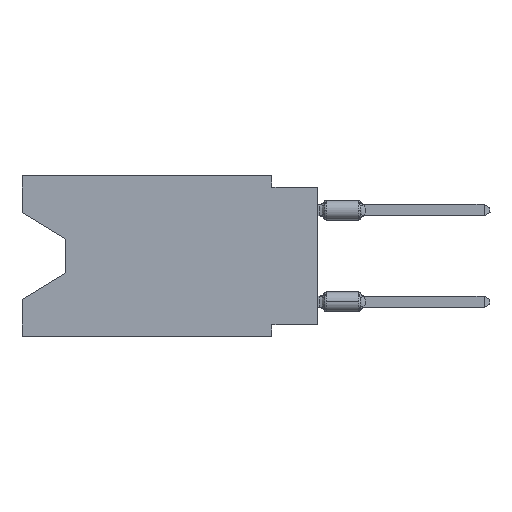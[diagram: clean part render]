
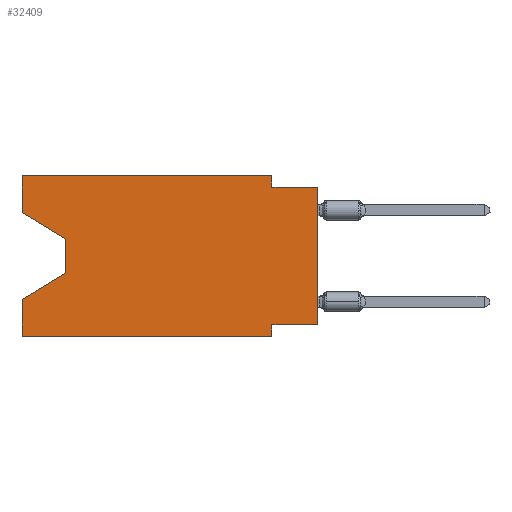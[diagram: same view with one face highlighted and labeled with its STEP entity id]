
A CAD part, left-side view. The second image highlights one B-rep face of the part: STEP entity #32409.
In plain terms, the highlighted planar face has unit normal (-1, 0, 0).
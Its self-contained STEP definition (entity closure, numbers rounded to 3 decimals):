
#1555 = VECTOR ( 'NONE', #13114, 1000. ) ;
#2127 = EDGE_CURVE ( 'NONE', #6122, #20296, #10588, .T. ) ;
#2424 = VECTOR ( 'NONE', #17949, 1000. ) ;
#2964 = ORIENTED_EDGE ( 'NONE', *, *, #2127, .T. ) ;
#3343 = CARTESIAN_POINT ( 'NONE',  ( 0., 16.383, 0. ) ) ;
#3591 = LINE ( 'NONE', #17284, #8170 ) ;
#3980 = EDGE_CURVE ( 'NONE', #21906, #12121, #20097, .T. ) ;
#5154 = VERTEX_POINT ( 'NONE', #24894 ) ;
#5401 = LINE ( 'NONE', #36167, #9045 ) ;
#5433 = ORIENTED_EDGE ( 'NONE', *, *, #13943, .T. ) ;
#6122 = VERTEX_POINT ( 'NONE', #23153 ) ;
#6613 = CARTESIAN_POINT ( 'NONE',  ( 0., 16.383, 0. ) ) ;
#7440 = DIRECTION ( 'NONE',  ( 0., -0.855, -0.519 ) ) ;
#7630 = VERTEX_POINT ( 'NONE', #41982 ) ;
#8170 = VECTOR ( 'NONE', #9881, 1000. ) ;
#8383 = CARTESIAN_POINT ( 'NONE',  ( 0., 13.97, -3.505 ) ) ;
#8502 = CARTESIAN_POINT ( 'NONE',  ( 0., 2.54, 0. ) ) ;
#9045 = VECTOR ( 'NONE', #22942, 1000. ) ;
#9091 = EDGE_CURVE ( 'NONE', #21906, #24335, #5401, .T. ) ;
#9234 = EDGE_LOOP ( 'NONE', ( #2964, #10664, #5433, #18871, #29404, #34020, #12532, #31172, #17175, #41282, #22954, #24127 ) ) ;
#9881 = DIRECTION ( 'NONE',  ( 0., -1., 0. ) ) ;
#10588 = LINE ( 'NONE', #38016, #40157 ) ;
#10664 = ORIENTED_EDGE ( 'NONE', *, *, #19713, .T. ) ;
#10834 = CARTESIAN_POINT ( 'NONE',  ( 0., 2.54, -8.255 ) ) ;
#10869 = AXIS2_PLACEMENT_3D ( 'NONE', #35671, #14783, #24690 ) ;
#11418 = FACE_OUTER_BOUND ( 'NONE', #9234, .T. ) ;
#11859 = DIRECTION ( 'NONE',  ( 0., 0., -1. ) ) ;
#12121 = VERTEX_POINT ( 'NONE', #19804 ) ;
#12532 = ORIENTED_EDGE ( 'NONE', *, *, #29474, .F. ) ;
#13114 = DIRECTION ( 'NONE',  ( 0., 0., 1. ) ) ;
#13943 = EDGE_CURVE ( 'NONE', #25953, #12121, #14110, .T. ) ;
#14110 = LINE ( 'NONE', #28056, #43841 ) ;
#14356 = LINE ( 'NONE', #28064, #2424 ) ;
#14604 = LINE ( 'NONE', #23880, #28732 ) ;
#14783 = DIRECTION ( 'NONE',  ( 1., 0., 0. ) ) ;
#14991 = VECTOR ( 'NONE', #36003, 1000. ) ;
#16098 = VECTOR ( 'NONE', #30619, 1000. ) ;
#17175 = ORIENTED_EDGE ( 'NONE', *, *, #29355, .F. ) ;
#17284 = CARTESIAN_POINT ( 'NONE',  ( 0., 0., -0.635 ) ) ;
#17919 = VERTEX_POINT ( 'NONE', #44196 ) ;
#17949 = DIRECTION ( 'NONE',  ( 0., 1., 0. ) ) ;
#18482 = LINE ( 'NONE', #8383, #14991 ) ;
#18871 = ORIENTED_EDGE ( 'NONE', *, *, #3980, .F. ) ;
#19713 = EDGE_CURVE ( 'NONE', #20296, #25953, #18482, .T. ) ;
#19804 = CARTESIAN_POINT ( 'NONE',  ( 0., 16.383, -6.852 ) ) ;
#20097 = LINE ( 'NONE', #6613, #1555 ) ;
#20296 = VERTEX_POINT ( 'NONE', #43381 ) ;
#20434 = LINE ( 'NONE', #3343, #37351 ) ;
#21488 = DIRECTION ( 'NONE',  ( 0., 0., 1. ) ) ;
#21906 = VERTEX_POINT ( 'NONE', #28738 ) ;
#22920 = EDGE_CURVE ( 'NONE', #6122, #33546, #14604, .T. ) ;
#22942 = DIRECTION ( 'NONE',  ( 0., -1., 0. ) ) ;
#22954 = ORIENTED_EDGE ( 'NONE', *, *, #23321, .F. ) ;
#23084 = VECTOR ( 'NONE', #21488, 1000. ) ;
#23153 = CARTESIAN_POINT ( 'NONE',  ( 0., 16.383, -2.038 ) ) ;
#23222 = CARTESIAN_POINT ( 'NONE',  ( 0., 16.383, 0. ) ) ;
#23321 = EDGE_CURVE ( 'NONE', #33546, #30967, #20434, .T. ) ;
#23689 = CARTESIAN_POINT ( 'NONE',  ( 0., 2.54, -8.89 ) ) ;
#23880 = CARTESIAN_POINT ( 'NONE',  ( 0., 16.383, 0. ) ) ;
#24127 = ORIENTED_EDGE ( 'NONE', *, *, #22920, .F. ) ;
#24335 = VERTEX_POINT ( 'NONE', #29056 ) ;
#24690 = DIRECTION ( 'NONE',  ( 0., 0., -1. ) ) ;
#24894 = CARTESIAN_POINT ( 'NONE',  ( 0., 0., -0.635 ) ) ;
#25081 = CARTESIAN_POINT ( 'NONE',  ( 0., 0., 0. ) ) ;
#25574 = LINE ( 'NONE', #8502, #38301 ) ;
#25953 = VERTEX_POINT ( 'NONE', #41848 ) ;
#28056 = CARTESIAN_POINT ( 'NONE',  ( 0., 13.97, -5.385 ) ) ;
#28064 = CARTESIAN_POINT ( 'NONE',  ( 0., 0., -8.255 ) ) ;
#28732 = VECTOR ( 'NONE', #42276, 1000. ) ;
#28734 = PLANE ( 'NONE',  #10869 ) ;
#28738 = CARTESIAN_POINT ( 'NONE',  ( 0., 16.383, -8.89 ) ) ;
#29056 = CARTESIAN_POINT ( 'NONE',  ( 0., 2.54, -8.89 ) ) ;
#29355 = EDGE_CURVE ( 'NONE', #7630, #5154, #3591, .T. ) ;
#29404 = ORIENTED_EDGE ( 'NONE', *, *, #9091, .T. ) ;
#29450 = EDGE_CURVE ( 'NONE', #30967, #7630, #25574, .T. ) ;
#29474 = EDGE_CURVE ( 'NONE', #17919, #44167, #14356, .T. ) ;
#30619 = DIRECTION ( 'NONE',  ( 0., 0., -1. ) ) ;
#30967 = VERTEX_POINT ( 'NONE', #43839 ) ;
#30990 = DIRECTION ( 'NONE',  ( 0., 0.855, -0.519 ) ) ;
#31172 = ORIENTED_EDGE ( 'NONE', *, *, #32789, .T. ) ;
#32409 = ADVANCED_FACE ( 'NONE', ( #11418 ), #28734, .F. ) ;
#32789 = EDGE_CURVE ( 'NONE', #17919, #5154, #35384, .T. ) ;
#33546 = VERTEX_POINT ( 'NONE', #23222 ) ;
#34020 = ORIENTED_EDGE ( 'NONE', *, *, #35601, .F. ) ;
#35384 = LINE ( 'NONE', #25081, #23084 ) ;
#35601 = EDGE_CURVE ( 'NONE', #44167, #24335, #40756, .T. ) ;
#35671 = CARTESIAN_POINT ( 'NONE',  ( 0., 16.383, 0. ) ) ;
#36003 = DIRECTION ( 'NONE',  ( 0., 0., -1. ) ) ;
#36167 = CARTESIAN_POINT ( 'NONE',  ( 0., 16.383, -8.89 ) ) ;
#37351 = VECTOR ( 'NONE', #44275, 1000. ) ;
#38016 = CARTESIAN_POINT ( 'NONE',  ( 0., 16.383, -2.038 ) ) ;
#38301 = VECTOR ( 'NONE', #11859, 1000. ) ;
#40157 = VECTOR ( 'NONE', #7440, 1000. ) ;
#40756 = LINE ( 'NONE', #23689, #16098 ) ;
#41282 = ORIENTED_EDGE ( 'NONE', *, *, #29450, .F. ) ;
#41848 = CARTESIAN_POINT ( 'NONE',  ( 0., 13.97, -5.385 ) ) ;
#41982 = CARTESIAN_POINT ( 'NONE',  ( 0., 2.54, -0.635 ) ) ;
#42276 = DIRECTION ( 'NONE',  ( 0., 0., 1. ) ) ;
#43381 = CARTESIAN_POINT ( 'NONE',  ( 0., 13.97, -3.505 ) ) ;
#43839 = CARTESIAN_POINT ( 'NONE',  ( 0., 2.54, 0. ) ) ;
#43841 = VECTOR ( 'NONE', #30990, 1000. ) ;
#44167 = VERTEX_POINT ( 'NONE', #10834 ) ;
#44196 = CARTESIAN_POINT ( 'NONE',  ( 0., 0., -8.255 ) ) ;
#44275 = DIRECTION ( 'NONE',  ( 0., -1., 0. ) ) ;
